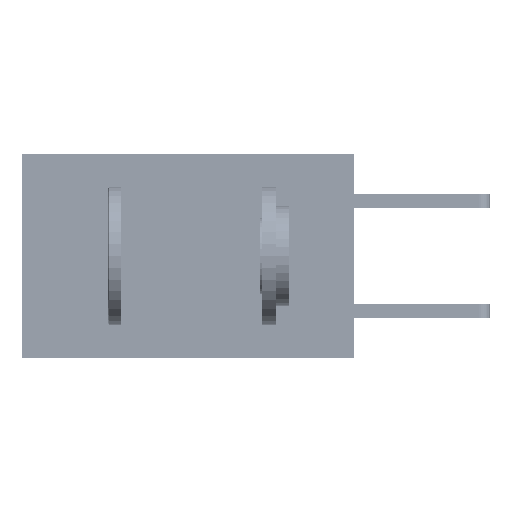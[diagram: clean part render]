
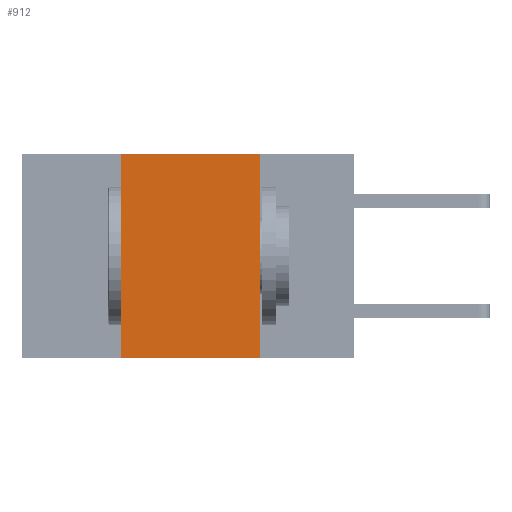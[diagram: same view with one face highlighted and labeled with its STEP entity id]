
A CAD part, left-side view. The second image highlights one B-rep face of the part: STEP entity #912.
In plain terms, the highlighted planar face has unit normal (-1, 0, 0).
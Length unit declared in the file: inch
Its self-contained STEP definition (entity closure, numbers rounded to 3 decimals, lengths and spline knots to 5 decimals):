
#123 = DIRECTION ( 'NONE',  ( 0., 0., -1. ) ) ;
#594 = VECTOR ( 'NONE', #42448, 39.37008 ) ;
#912 = ADVANCED_FACE ( 'NONE', ( #5332 ), #8739, .F. ) ;
#1449 = DIRECTION ( 'NONE',  ( 0., 0., 1. ) ) ;
#1777 = VERTEX_POINT ( 'NONE', #30822 ) ;
#3652 = VECTOR ( 'NONE', #12079, 39.37008 ) ;
#4783 = EDGE_CURVE ( 'NONE', #9940, #45281, #30365, .T. ) ;
#5332 = FACE_OUTER_BOUND ( 'NONE', #22222, .T. ) ;
#8739 = PLANE ( 'NONE',  #34196 ) ;
#9940 = VERTEX_POINT ( 'NONE', #15958 ) ;
#11625 = VECTOR ( 'NONE', #1449, 39.37008 ) ;
#11847 = DIRECTION ( 'NONE',  ( 0., -1., 0. ) ) ;
#11953 = EDGE_CURVE ( 'NONE', #1777, #43537, #22417, .T. ) ;
#12079 = DIRECTION ( 'NONE',  ( 0., 0., -1. ) ) ;
#15958 = CARTESIAN_POINT ( 'NONE',  ( 0., 0.17, 0. ) ) ;
#16707 = EDGE_CURVE ( 'NONE', #1777, #45281, #19696, .T. ) ;
#17063 = EDGE_CURVE ( 'NONE', #43537, #9940, #43105, .T. ) ;
#17066 = ORIENTED_EDGE ( 'NONE', *, *, #4783, .F. ) ;
#19696 = LINE ( 'NONE', #32065, #52031 ) ;
#22222 = EDGE_LOOP ( 'NONE', ( #17066, #33212, #42391, #32408 ) ) ;
#22417 = LINE ( 'NONE', #25942, #11625 ) ;
#25942 = CARTESIAN_POINT ( 'NONE',  ( 0., 0.42, 0. ) ) ;
#29993 = CARTESIAN_POINT ( 'NONE',  ( 0., 0.17, -0.37 ) ) ;
#30365 = LINE ( 'NONE', #32472, #3652 ) ;
#30822 = CARTESIAN_POINT ( 'NONE',  ( 0., 0.42, -0.37 ) ) ;
#32065 = CARTESIAN_POINT ( 'NONE',  ( 0., 0.6, -0.37 ) ) ;
#32408 = ORIENTED_EDGE ( 'NONE', *, *, #16707, .T. ) ;
#32472 = CARTESIAN_POINT ( 'NONE',  ( 0., 0.17, 0. ) ) ;
#33101 = CARTESIAN_POINT ( 'NONE',  ( 0., 0.6, 0. ) ) ;
#33212 = ORIENTED_EDGE ( 'NONE', *, *, #17063, .F. ) ;
#34196 = AXIS2_PLACEMENT_3D ( 'NONE', #33101, #37149, #123 ) ;
#37149 = DIRECTION ( 'NONE',  ( 1., 0., 0. ) ) ;
#42391 = ORIENTED_EDGE ( 'NONE', *, *, #11953, .F. ) ;
#42448 = DIRECTION ( 'NONE',  ( 0., -1., 0. ) ) ;
#43105 = LINE ( 'NONE', #50635, #594 ) ;
#43537 = VERTEX_POINT ( 'NONE', #47210 ) ;
#45281 = VERTEX_POINT ( 'NONE', #29993 ) ;
#47210 = CARTESIAN_POINT ( 'NONE',  ( 0., 0.42, 0. ) ) ;
#50635 = CARTESIAN_POINT ( 'NONE',  ( 0., 0.6, 0. ) ) ;
#52031 = VECTOR ( 'NONE', #11847, 39.37008 ) ;
